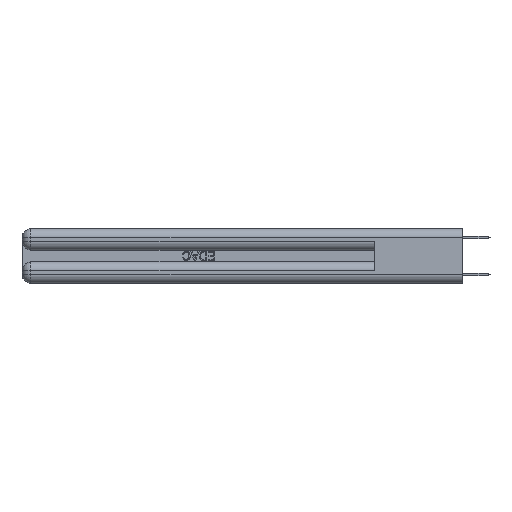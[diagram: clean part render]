
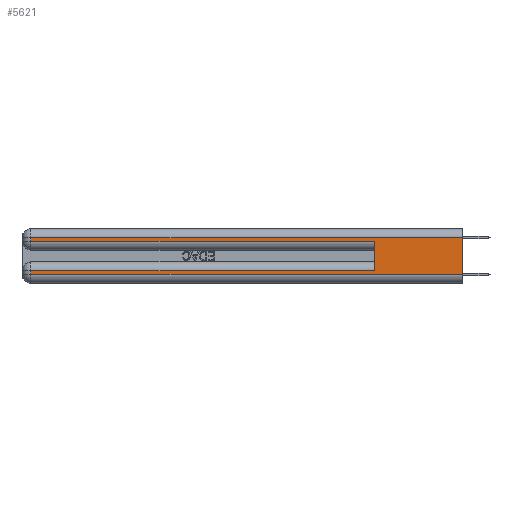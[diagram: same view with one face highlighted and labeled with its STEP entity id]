
A CAD part, left-side view. The second image highlights one B-rep face of the part: STEP entity #5621.
In plain terms, the highlighted planar face has unit normal (-1, 0, 0).
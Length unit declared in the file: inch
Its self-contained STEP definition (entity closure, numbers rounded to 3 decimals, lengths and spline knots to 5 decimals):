
#57 = VERTEX_POINT ( 'NONE', #26487 ) ;
#140 = DIRECTION ( 'NONE',  ( 0., 0., -1. ) ) ;
#693 = DIRECTION ( 'NONE',  ( 1., 0., 0. ) ) ;
#1427 = ORIENTED_EDGE ( 'NONE', *, *, #4815, .T. ) ;
#1545 = VERTEX_POINT ( 'NONE', #19877 ) ;
#2337 = VECTOR ( 'NONE', #9076, 39.37008 ) ;
#2420 = CARTESIAN_POINT ( 'NONE',  ( 0., 0., 0.06 ) ) ;
#2430 = FACE_OUTER_BOUND ( 'NONE', #15207, .T. ) ;
#2576 = AXIS2_PLACEMENT_3D ( 'NONE', #26582, #693, #12074 ) ;
#3420 = CARTESIAN_POINT ( 'NONE',  ( 0., 2.94, 0.37 ) ) ;
#3509 = EDGE_CURVE ( 'NONE', #10349, #26977, #7297, .T. ) ;
#3848 = ORIENTED_EDGE ( 'NONE', *, *, #3509, .T. ) ;
#4616 = VECTOR ( 'NONE', #13946, 39.37008 ) ;
#4815 = EDGE_CURVE ( 'NONE', #1545, #11008, #8558, .T. ) ;
#5251 = ORIENTED_EDGE ( 'NONE', *, *, #12916, .T. ) ;
#5621 = ADVANCED_FACE ( 'NONE', ( #2430 ), #10176, .F. ) ;
#6675 = CARTESIAN_POINT ( 'NONE',  ( 0., 0., 0.085 ) ) ;
#6723 = LINE ( 'NONE', #16617, #13940 ) ;
#7297 = LINE ( 'NONE', #24002, #24908 ) ;
#7735 = CARTESIAN_POINT ( 'NONE',  ( 0., 0., 0.31 ) ) ;
#8558 = LINE ( 'NONE', #3420, #18047 ) ;
#8929 = ORIENTED_EDGE ( 'NONE', *, *, #10866, .F. ) ;
#9076 = DIRECTION ( 'NONE',  ( 0., -1., 0. ) ) ;
#10176 = PLANE ( 'NONE',  #2576 ) ;
#10349 = VERTEX_POINT ( 'NONE', #25174 ) ;
#10573 = DIRECTION ( 'NONE',  ( 0., 0., -1. ) ) ;
#10866 = EDGE_CURVE ( 'NONE', #27944, #14687, #17851, .T. ) ;
#11008 = VERTEX_POINT ( 'NONE', #18946 ) ;
#12074 = DIRECTION ( 'NONE',  ( 0., 0., -1. ) ) ;
#12916 = EDGE_CURVE ( 'NONE', #29061, #1545, #15965, .T. ) ;
#13770 = LINE ( 'NONE', #17964, #29225 ) ;
#13940 = VECTOR ( 'NONE', #18815, 39.37008 ) ;
#13946 = DIRECTION ( 'NONE',  ( 0., 1., 0. ) ) ;
#14687 = VERTEX_POINT ( 'NONE', #2420 ) ;
#15207 = EDGE_LOOP ( 'NONE', ( #8929, #21782, #3848, #20629, #30152, #5251, #1427, #17302 ) ) ;
#15965 = LINE ( 'NONE', #6675, #4616 ) ;
#16134 = EDGE_CURVE ( 'NONE', #26977, #57, #29477, .T. ) ;
#16138 = DIRECTION ( 'NONE',  ( 0., 0., -1. ) ) ;
#16617 = CARTESIAN_POINT ( 'NONE',  ( 0., 0., 0.31 ) ) ;
#17302 = ORIENTED_EDGE ( 'NONE', *, *, #19933, .T. ) ;
#17851 = LINE ( 'NONE', #26030, #18205 ) ;
#17964 = CARTESIAN_POINT ( 'NONE',  ( 0., 0.6, 0.145 ) ) ;
#18047 = VECTOR ( 'NONE', #10573, 39.37008 ) ;
#18205 = VECTOR ( 'NONE', #16138, 39.37008 ) ;
#18815 = DIRECTION ( 'NONE',  ( 0., 1., 0. ) ) ;
#18946 = CARTESIAN_POINT ( 'NONE',  ( 0., 2.94, 0.06 ) ) ;
#19877 = CARTESIAN_POINT ( 'NONE',  ( 0., 2.94, 0.085 ) ) ;
#19933 = EDGE_CURVE ( 'NONE', #11008, #14687, #20837, .T. ) ;
#20232 = DIRECTION ( 'NONE',  ( 0., -1., 0. ) ) ;
#20629 = ORIENTED_EDGE ( 'NONE', *, *, #16134, .T. ) ;
#20837 = LINE ( 'NONE', #30220, #2337 ) ;
#21782 = ORIENTED_EDGE ( 'NONE', *, *, #29537, .T. ) ;
#23240 = DIRECTION ( 'NONE',  ( 0., 0., 1. ) ) ;
#24002 = CARTESIAN_POINT ( 'NONE',  ( 0., 2.94, 0.37 ) ) ;
#24899 = VECTOR ( 'NONE', #20232, 39.37008 ) ;
#24908 = VECTOR ( 'NONE', #140, 39.37008 ) ;
#25174 = CARTESIAN_POINT ( 'NONE',  ( 0., 2.94, 0.31 ) ) ;
#26030 = CARTESIAN_POINT ( 'NONE',  ( 0., 0., 0.37 ) ) ;
#26487 = CARTESIAN_POINT ( 'NONE',  ( 0., 0.6, 0.285 ) ) ;
#26526 = CARTESIAN_POINT ( 'NONE',  ( 0., 2.94, 0.285 ) ) ;
#26582 = CARTESIAN_POINT ( 'NONE',  ( 0., 0., 0.37 ) ) ;
#26977 = VERTEX_POINT ( 'NONE', #26526 ) ;
#27944 = VERTEX_POINT ( 'NONE', #7735 ) ;
#29061 = VERTEX_POINT ( 'NONE', #29636 ) ;
#29176 = CARTESIAN_POINT ( 'NONE',  ( 0., 0., 0.285 ) ) ;
#29225 = VECTOR ( 'NONE', #23240, 39.37008 ) ;
#29477 = LINE ( 'NONE', #29176, #24899 ) ;
#29537 = EDGE_CURVE ( 'NONE', #27944, #10349, #6723, .T. ) ;
#29636 = CARTESIAN_POINT ( 'NONE',  ( 0., 0.6, 0.085 ) ) ;
#29900 = EDGE_CURVE ( 'NONE', #29061, #57, #13770, .T. ) ;
#30152 = ORIENTED_EDGE ( 'NONE', *, *, #29900, .F. ) ;
#30220 = CARTESIAN_POINT ( 'NONE',  ( 0., 0., 0.06 ) ) ;
